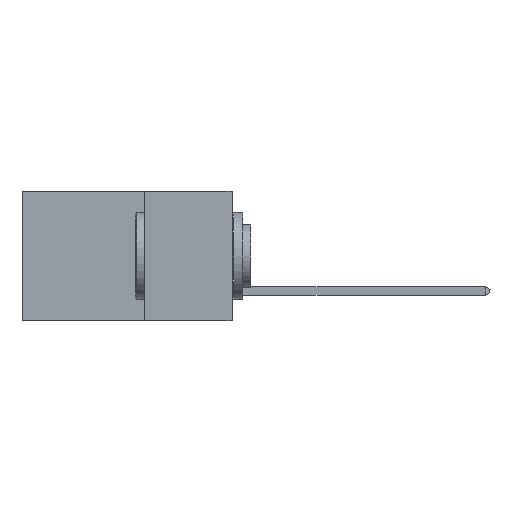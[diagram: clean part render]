
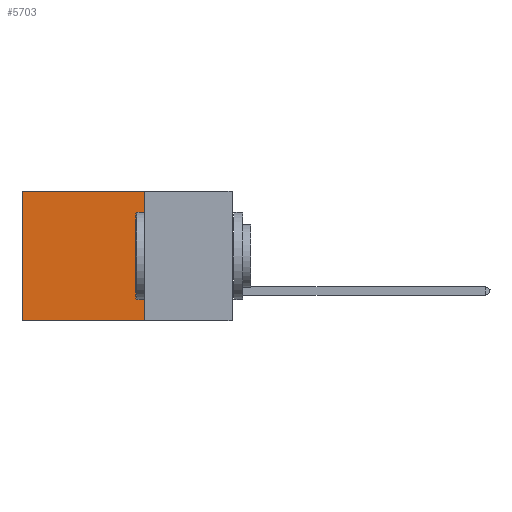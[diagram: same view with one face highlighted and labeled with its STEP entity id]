
A CAD part, left-side view. The second image highlights one B-rep face of the part: STEP entity #5703.
In plain terms, the highlighted planar face has unit normal (-1, 0, 0).
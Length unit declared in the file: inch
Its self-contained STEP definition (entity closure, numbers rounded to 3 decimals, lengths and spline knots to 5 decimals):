
#106 = CARTESIAN_POINT ( 'NONE',  ( 0.2875, 0.25, 0. ) ) ;
#359 = CARTESIAN_POINT ( 'NONE',  ( 0.2875, 0.25, -0.37 ) ) ;
#414 = ORIENTED_EDGE ( 'NONE', *, *, #2734, .F. ) ;
#551 = DIRECTION ( 'NONE',  ( 0., 0., -1. ) ) ;
#1155 = DIRECTION ( 'NONE',  ( 0., 0., -1. ) ) ;
#1708 = CARTESIAN_POINT ( 'NONE',  ( 0.2875, 0.25, -0.37 ) ) ;
#2456 = LINE ( 'NONE', #10522, #17372 ) ;
#2670 = LINE ( 'NONE', #359, #8308 ) ;
#2734 = EDGE_CURVE ( 'NONE', #12989, #6088, #2670, .T. ) ;
#3007 = VERTEX_POINT ( 'NONE', #106 ) ;
#3381 = FACE_OUTER_BOUND ( 'NONE', #10689, .T. ) ;
#4198 = ORIENTED_EDGE ( 'NONE', *, *, #6728, .T. ) ;
#4548 = AXIS2_PLACEMENT_3D ( 'NONE', #12740, #17083, #8434 ) ;
#5703 = ADVANCED_FACE ( 'NONE', ( #3381 ), #6996, .F. ) ;
#5865 = VECTOR ( 'NONE', #14705, 39.37008 ) ;
#6088 = VERTEX_POINT ( 'NONE', #16782 ) ;
#6728 = EDGE_CURVE ( 'NONE', #7912, #6088, #2456, .T. ) ;
#6788 = LINE ( 'NONE', #13262, #5865 ) ;
#6996 = PLANE ( 'NONE',  #4548 ) ;
#7912 = VERTEX_POINT ( 'NONE', #13483 ) ;
#8308 = VECTOR ( 'NONE', #16263, 39.37008 ) ;
#8434 = DIRECTION ( 'NONE',  ( 0., 0., -1. ) ) ;
#9136 = ORIENTED_EDGE ( 'NONE', *, *, #15403, .F. ) ;
#9711 = CARTESIAN_POINT ( 'NONE',  ( 0.2875, 0.25, 0. ) ) ;
#10522 = CARTESIAN_POINT ( 'NONE',  ( 0.2875, 0.6, 0. ) ) ;
#10689 = EDGE_LOOP ( 'NONE', ( #4198, #414, #9136, #12094 ) ) ;
#11462 = VECTOR ( 'NONE', #1155, 39.37008 ) ;
#12094 = ORIENTED_EDGE ( 'NONE', *, *, #12980, .T. ) ;
#12740 = CARTESIAN_POINT ( 'NONE',  ( 0.2875, 0.25, 0. ) ) ;
#12980 = EDGE_CURVE ( 'NONE', #3007, #7912, #6788, .T. ) ;
#12989 = VERTEX_POINT ( 'NONE', #1708 ) ;
#13262 = CARTESIAN_POINT ( 'NONE',  ( 0.2875, 0.25, 0. ) ) ;
#13483 = CARTESIAN_POINT ( 'NONE',  ( 0.2875, 0.6, 0. ) ) ;
#14705 = DIRECTION ( 'NONE',  ( 0., 1., 0. ) ) ;
#15403 = EDGE_CURVE ( 'NONE', #3007, #12989, #15966, .T. ) ;
#15966 = LINE ( 'NONE', #9711, #11462 ) ;
#16263 = DIRECTION ( 'NONE',  ( 0., 1., 0. ) ) ;
#16782 = CARTESIAN_POINT ( 'NONE',  ( 0.2875, 0.6, -0.37 ) ) ;
#17083 = DIRECTION ( 'NONE',  ( 1., 0., 0. ) ) ;
#17372 = VECTOR ( 'NONE', #551, 39.37008 ) ;
